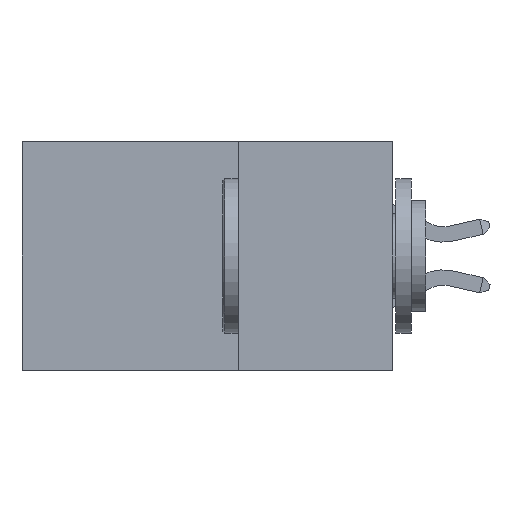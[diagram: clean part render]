
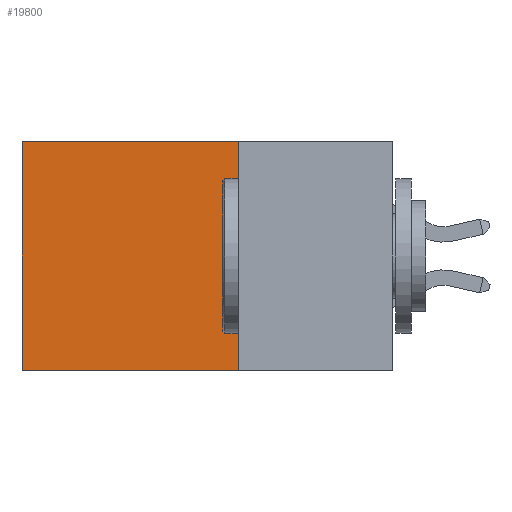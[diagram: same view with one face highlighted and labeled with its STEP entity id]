
A CAD part, left-side view. The second image highlights one B-rep face of the part: STEP entity #19800.
In plain terms, the highlighted planar face has unit normal (-1, 0, 0).
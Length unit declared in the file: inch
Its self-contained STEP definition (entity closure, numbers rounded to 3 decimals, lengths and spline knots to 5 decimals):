
#137 = ORIENTED_EDGE ( 'NONE', *, *, #20081, .F. ) ;
#1397 = DIRECTION ( 'NONE',  ( 0., 0., -1. ) ) ;
#1662 = VECTOR ( 'NONE', #25160, 39.37008 ) ;
#3290 = VECTOR ( 'NONE', #31244, 39.37008 ) ;
#3844 = ORIENTED_EDGE ( 'NONE', *, *, #30796, .T. ) ;
#4576 = VERTEX_POINT ( 'NONE', #7319 ) ;
#7301 = CARTESIAN_POINT ( 'NONE',  ( 0.2875, 0.25, -0.37 ) ) ;
#7319 = CARTESIAN_POINT ( 'NONE',  ( 0.2875, 0.6, -0.37 ) ) ;
#8661 = PLANE ( 'NONE',  #16495 ) ;
#9289 = EDGE_LOOP ( 'NONE', ( #3844, #25129, #137, #20563 ) ) ;
#10644 = CARTESIAN_POINT ( 'NONE',  ( 0.2875, 0.25, 0. ) ) ;
#10993 = CARTESIAN_POINT ( 'NONE',  ( 0.2875, 0.25, -0.37 ) ) ;
#11554 = VERTEX_POINT ( 'NONE', #24294 ) ;
#11883 = LINE ( 'NONE', #30284, #1662 ) ;
#12215 = CARTESIAN_POINT ( 'NONE',  ( 0.2875, 0.25, 0. ) ) ;
#13623 = LINE ( 'NONE', #7301, #27280 ) ;
#14223 = DIRECTION ( 'NONE',  ( 0., 1., 0. ) ) ;
#15812 = DIRECTION ( 'NONE',  ( 1., 0., 0. ) ) ;
#16495 = AXIS2_PLACEMENT_3D ( 'NONE', #20560, #15812, #1397 ) ;
#17212 = LINE ( 'NONE', #12215, #3290 ) ;
#19800 = ADVANCED_FACE ( 'NONE', ( #26402 ), #8661, .F. ) ;
#20081 = EDGE_CURVE ( 'NONE', #22271, #24905, #17212, .T. ) ;
#20560 = CARTESIAN_POINT ( 'NONE',  ( 0.2875, 0.25, 0. ) ) ;
#20563 = ORIENTED_EDGE ( 'NONE', *, *, #22129, .T. ) ;
#22129 = EDGE_CURVE ( 'NONE', #22271, #11554, #11883, .T. ) ;
#22271 = VERTEX_POINT ( 'NONE', #10644 ) ;
#23220 = CARTESIAN_POINT ( 'NONE',  ( 0.2875, 0.6, 0. ) ) ;
#24294 = CARTESIAN_POINT ( 'NONE',  ( 0.2875, 0.6, 0. ) ) ;
#24416 = LINE ( 'NONE', #23220, #25213 ) ;
#24905 = VERTEX_POINT ( 'NONE', #10993 ) ;
#25129 = ORIENTED_EDGE ( 'NONE', *, *, #27915, .F. ) ;
#25160 = DIRECTION ( 'NONE',  ( 0., 1., 0. ) ) ;
#25213 = VECTOR ( 'NONE', #30466, 39.37008 ) ;
#26402 = FACE_OUTER_BOUND ( 'NONE', #9289, .T. ) ;
#27280 = VECTOR ( 'NONE', #14223, 39.37008 ) ;
#27915 = EDGE_CURVE ( 'NONE', #24905, #4576, #13623, .T. ) ;
#30284 = CARTESIAN_POINT ( 'NONE',  ( 0.2875, 0.25, 0. ) ) ;
#30466 = DIRECTION ( 'NONE',  ( 0., 0., -1. ) ) ;
#30796 = EDGE_CURVE ( 'NONE', #11554, #4576, #24416, .T. ) ;
#31244 = DIRECTION ( 'NONE',  ( 0., 0., -1. ) ) ;
